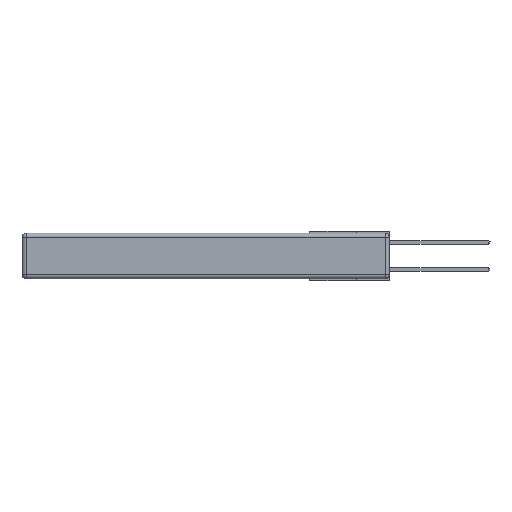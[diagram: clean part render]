
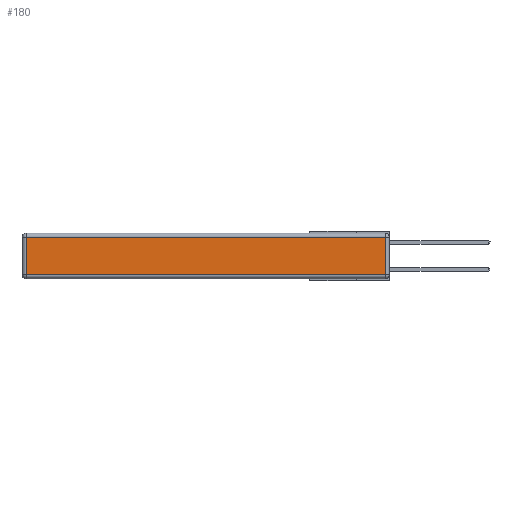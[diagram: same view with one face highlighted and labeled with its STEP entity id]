
A CAD part, left-side view. The second image highlights one B-rep face of the part: STEP entity #180.
In plain terms, the highlighted planar face has unit normal (-1, 0, 0).
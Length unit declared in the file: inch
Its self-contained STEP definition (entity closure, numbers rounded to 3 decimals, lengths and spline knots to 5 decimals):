
#163 = CARTESIAN_POINT ( 'NONE',  ( 0., 2.72, -0.313 ) ) ;
#180 = ADVANCED_FACE ( 'NONE', ( #1910 ), #9349, .T. ) ;
#321 = CARTESIAN_POINT ( 'NONE',  ( 0., 0.03, -0.03 ) ) ;
#781 = EDGE_CURVE ( 'NONE', #9433, #2399, #8011, .T. ) ;
#851 = VECTOR ( 'NONE', #7419, 39.37008 ) ;
#933 = EDGE_LOOP ( 'NONE', ( #12565, #8711, #6365, #5784 ) ) ;
#1761 = VERTEX_POINT ( 'NONE', #10331 ) ;
#1805 = CARTESIAN_POINT ( 'NONE',  ( 0., 2.72, -0.343 ) ) ;
#1889 = EDGE_CURVE ( 'NONE', #11477, #9433, #7967, .T. ) ;
#1910 = FACE_OUTER_BOUND ( 'NONE', #933, .T. ) ;
#2080 = EDGE_CURVE ( 'NONE', #2399, #1761, #2196, .T. ) ;
#2196 = LINE ( 'NONE', #14762, #13121 ) ;
#2318 = DIRECTION ( 'NONE',  ( 0., 0., 1. ) ) ;
#2399 = VERTEX_POINT ( 'NONE', #163 ) ;
#3129 = LINE ( 'NONE', #11934, #851 ) ;
#5784 = ORIENTED_EDGE ( 'NONE', *, *, #781, .T. ) ;
#6365 = ORIENTED_EDGE ( 'NONE', *, *, #1889, .T. ) ;
#6659 = DIRECTION ( 'NONE',  ( 0., 0., -1. ) ) ;
#7265 = AXIS2_PLACEMENT_3D ( 'NONE', #11700, #10450, #2318 ) ;
#7419 = DIRECTION ( 'NONE',  ( 0., 0., 1. ) ) ;
#7518 = DIRECTION ( 'NONE',  ( 0., 1., 0. ) ) ;
#7967 = LINE ( 'NONE', #8448, #10359 ) ;
#8011 = LINE ( 'NONE', #1805, #14843 ) ;
#8448 = CARTESIAN_POINT ( 'NONE',  ( 0., 2.75, -0.03 ) ) ;
#8711 = ORIENTED_EDGE ( 'NONE', *, *, #14391, .T. ) ;
#9349 = PLANE ( 'NONE',  #7265 ) ;
#9433 = VERTEX_POINT ( 'NONE', #11843 ) ;
#10331 = CARTESIAN_POINT ( 'NONE',  ( 0., 0.03, -0.313 ) ) ;
#10359 = VECTOR ( 'NONE', #7518, 39.37008 ) ;
#10450 = DIRECTION ( 'NONE',  ( -1., 0., 0. ) ) ;
#11477 = VERTEX_POINT ( 'NONE', #321 ) ;
#11700 = CARTESIAN_POINT ( 'NONE',  ( 0., 0., -0.343 ) ) ;
#11843 = CARTESIAN_POINT ( 'NONE',  ( 0., 2.72, -0.03 ) ) ;
#11934 = CARTESIAN_POINT ( 'NONE',  ( 0., 0.03, -0.343 ) ) ;
#12394 = DIRECTION ( 'NONE',  ( 0., -1., 0. ) ) ;
#12565 = ORIENTED_EDGE ( 'NONE', *, *, #2080, .T. ) ;
#13121 = VECTOR ( 'NONE', #12394, 39.37008 ) ;
#14391 = EDGE_CURVE ( 'NONE', #1761, #11477, #3129, .T. ) ;
#14762 = CARTESIAN_POINT ( 'NONE',  ( 0., 0., -0.313 ) ) ;
#14843 = VECTOR ( 'NONE', #6659, 39.37008 ) ;
